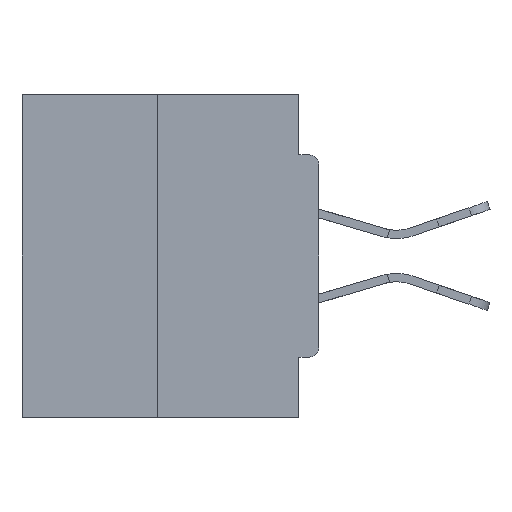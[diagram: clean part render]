
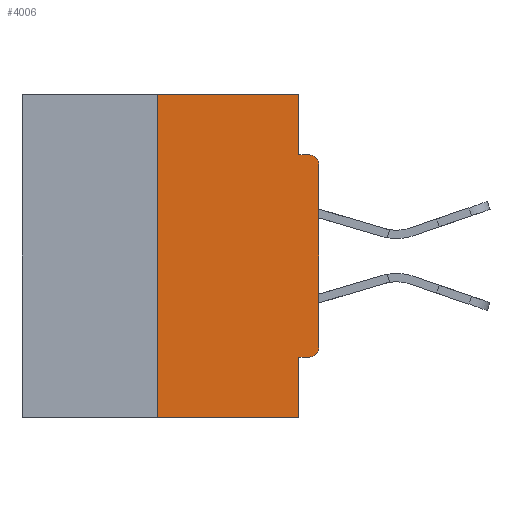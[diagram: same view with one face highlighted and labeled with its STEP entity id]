
A CAD part, left-side view. The second image highlights one B-rep face of the part: STEP entity #4006.
In plain terms, the highlighted planar face has unit normal (-1, 0, 0).
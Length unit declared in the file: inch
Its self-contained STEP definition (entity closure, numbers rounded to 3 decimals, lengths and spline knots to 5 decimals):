
#1682 = EDGE_LOOP ( 'NONE', ( #26818, #30332, #19755, #8587, #32802, #30401, #20944, #17197, #33503, #21597 ) ) ;
#2103 = CARTESIAN_POINT ( 'NONE',  ( 0., 0.015, -0.4065 ) ) ;
#2354 = CARTESIAN_POINT ( 'NONE',  ( 0., 0.46, 0. ) ) ;
#2990 = VERTEX_POINT ( 'NONE', #33545 ) ;
#3321 = LINE ( 'NONE', #27803, #31733 ) ;
#3416 = LINE ( 'NONE', #15879, #33527 ) ;
#4006 = ADVANCED_FACE ( 'NONE', ( #19044 ), #7890, .F. ) ;
#4613 = AXIS2_PLACEMENT_3D ( 'NONE', #11050, #24240, #26565 ) ;
#4877 = CARTESIAN_POINT ( 'NONE',  ( 0., 0., -0.1085 ) ) ;
#5151 = LINE ( 'NONE', #12844, #25606 ) ;
#5607 = VERTEX_POINT ( 'NONE', #32249 ) ;
#6781 = CIRCLE ( 'NONE', #22518, 0.015 ) ;
#7766 = VERTEX_POINT ( 'NONE', #2103 ) ;
#7890 = PLANE ( 'NONE',  #4613 ) ;
#8587 = ORIENTED_EDGE ( 'NONE', *, *, #27853, .F. ) ;
#8728 = DIRECTION ( 'NONE',  ( 0., -1., 0. ) ) ;
#8836 = VECTOR ( 'NONE', #18271, 39.37008 ) ;
#10085 = CARTESIAN_POINT ( 'NONE',  ( 0., 0.031, -0.5 ) ) ;
#10302 = EDGE_CURVE ( 'NONE', #12102, #32961, #20164, .T. ) ;
#11050 = CARTESIAN_POINT ( 'NONE',  ( 0., 0.46, 0. ) ) ;
#11490 = DIRECTION ( 'NONE',  ( 0., 0., -1. ) ) ;
#11613 = DIRECTION ( 'NONE',  ( -1., 0., 0. ) ) ;
#11644 = CARTESIAN_POINT ( 'NONE',  ( 0., 0.25, -0.5 ) ) ;
#12102 = VERTEX_POINT ( 'NONE', #17609 ) ;
#12844 = CARTESIAN_POINT ( 'NONE',  ( 0., 0.031, 0. ) ) ;
#13689 = DIRECTION ( 'NONE',  ( 0., 0., -1. ) ) ;
#13882 = EDGE_CURVE ( 'NONE', #32961, #24329, #6781, .T. ) ;
#14667 = DIRECTION ( 'NONE',  ( 0., 0., -1. ) ) ;
#14806 = EDGE_CURVE ( 'NONE', #7766, #34555, #3321, .T. ) ;
#14963 = EDGE_CURVE ( 'NONE', #7766, #12102, #15861, .T. ) ;
#15180 = VECTOR ( 'NONE', #11490, 39.37008 ) ;
#15861 = CIRCLE ( 'NONE', #25863, 0.015 ) ;
#15872 = CARTESIAN_POINT ( 'NONE',  ( 0., 0.015, -0.3915 ) ) ;
#15879 = CARTESIAN_POINT ( 'NONE',  ( 0., 0., -0.0935 ) ) ;
#17197 = ORIENTED_EDGE ( 'NONE', *, *, #13882, .T. ) ;
#17420 = CARTESIAN_POINT ( 'NONE',  ( 0., 0.25, 0. ) ) ;
#17609 = CARTESIAN_POINT ( 'NONE',  ( 0., 0., -0.3915 ) ) ;
#18271 = DIRECTION ( 'NONE',  ( 0., -1., 0. ) ) ;
#18951 = EDGE_CURVE ( 'NONE', #5607, #2990, #5151, .T. ) ;
#18981 = VERTEX_POINT ( 'NONE', #10085 ) ;
#19034 = CARTESIAN_POINT ( 'NONE',  ( 0., 0.25, 0. ) ) ;
#19044 = FACE_OUTER_BOUND ( 'NONE', #1682, .T. ) ;
#19343 = CARTESIAN_POINT ( 'NONE',  ( 0., 0.031, -0.5 ) ) ;
#19727 = LINE ( 'NONE', #30013, #25959 ) ;
#19755 = ORIENTED_EDGE ( 'NONE', *, *, #28711, .T. ) ;
#19789 = EDGE_CURVE ( 'NONE', #27070, #5607, #20153, .T. ) ;
#20153 = LINE ( 'NONE', #2354, #8836 ) ;
#20164 = LINE ( 'NONE', #23093, #21810 ) ;
#20216 = LINE ( 'NONE', #19343, #15180 ) ;
#20944 = ORIENTED_EDGE ( 'NONE', *, *, #10302, .T. ) ;
#21115 = DIRECTION ( 'NONE',  ( 0., -1., 0. ) ) ;
#21597 = ORIENTED_EDGE ( 'NONE', *, *, #18951, .F. ) ;
#21810 = VECTOR ( 'NONE', #31137, 39.37008 ) ;
#21850 = DIRECTION ( 'NONE',  ( -1., 0., 0. ) ) ;
#21919 = VERTEX_POINT ( 'NONE', #11644 ) ;
#22518 = AXIS2_PLACEMENT_3D ( 'NONE', #32510, #21850, #13689 ) ;
#23093 = CARTESIAN_POINT ( 'NONE',  ( 0., 0., 0. ) ) ;
#24240 = DIRECTION ( 'NONE',  ( 1., 0., 0. ) ) ;
#24329 = VERTEX_POINT ( 'NONE', #26884 ) ;
#25606 = VECTOR ( 'NONE', #34344, 39.37008 ) ;
#25863 = AXIS2_PLACEMENT_3D ( 'NONE', #15872, #11613, #14667 ) ;
#25959 = VECTOR ( 'NONE', #8728, 39.37008 ) ;
#26565 = DIRECTION ( 'NONE',  ( 0., 0., -1. ) ) ;
#26815 = DIRECTION ( 'NONE',  ( 0., 0., 1. ) ) ;
#26818 = ORIENTED_EDGE ( 'NONE', *, *, #19789, .F. ) ;
#26884 = CARTESIAN_POINT ( 'NONE',  ( 0., 0.015, -0.0935 ) ) ;
#27070 = VERTEX_POINT ( 'NONE', #17420 ) ;
#27558 = DIRECTION ( 'NONE',  ( 0., 1., 0. ) ) ;
#27803 = CARTESIAN_POINT ( 'NONE',  ( 0., 0., -0.4065 ) ) ;
#27853 = EDGE_CURVE ( 'NONE', #34555, #18981, #20216, .T. ) ;
#28391 = VECTOR ( 'NONE', #26815, 39.37008 ) ;
#28543 = EDGE_CURVE ( 'NONE', #2990, #24329, #3416, .T. ) ;
#28711 = EDGE_CURVE ( 'NONE', #21919, #18981, #19727, .T. ) ;
#30013 = CARTESIAN_POINT ( 'NONE',  ( 0., 0.46, -0.5 ) ) ;
#30332 = ORIENTED_EDGE ( 'NONE', *, *, #34322, .F. ) ;
#30401 = ORIENTED_EDGE ( 'NONE', *, *, #14963, .T. ) ;
#31137 = DIRECTION ( 'NONE',  ( 0., 0., 1. ) ) ;
#31730 = LINE ( 'NONE', #19034, #28391 ) ;
#31733 = VECTOR ( 'NONE', #27558, 39.37008 ) ;
#32249 = CARTESIAN_POINT ( 'NONE',  ( 0., 0.031, 0. ) ) ;
#32510 = CARTESIAN_POINT ( 'NONE',  ( 0., 0.015, -0.1085 ) ) ;
#32802 = ORIENTED_EDGE ( 'NONE', *, *, #14806, .F. ) ;
#32961 = VERTEX_POINT ( 'NONE', #4877 ) ;
#33057 = CARTESIAN_POINT ( 'NONE',  ( 0., 0.031, -0.4065 ) ) ;
#33503 = ORIENTED_EDGE ( 'NONE', *, *, #28543, .F. ) ;
#33527 = VECTOR ( 'NONE', #21115, 39.37008 ) ;
#33545 = CARTESIAN_POINT ( 'NONE',  ( 0., 0.031, -0.0935 ) ) ;
#34322 = EDGE_CURVE ( 'NONE', #21919, #27070, #31730, .T. ) ;
#34344 = DIRECTION ( 'NONE',  ( 0., 0., -1. ) ) ;
#34555 = VERTEX_POINT ( 'NONE', #33057 ) ;
